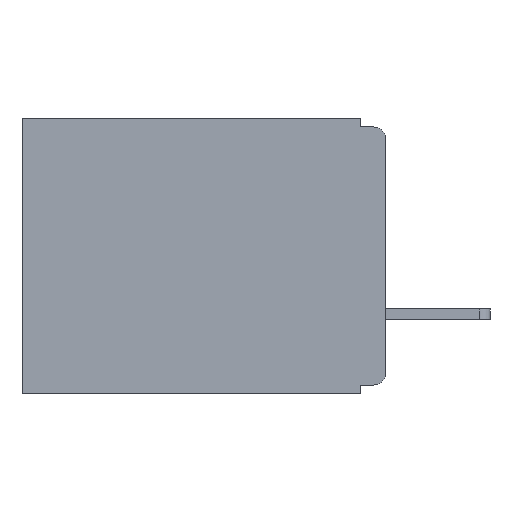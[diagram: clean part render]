
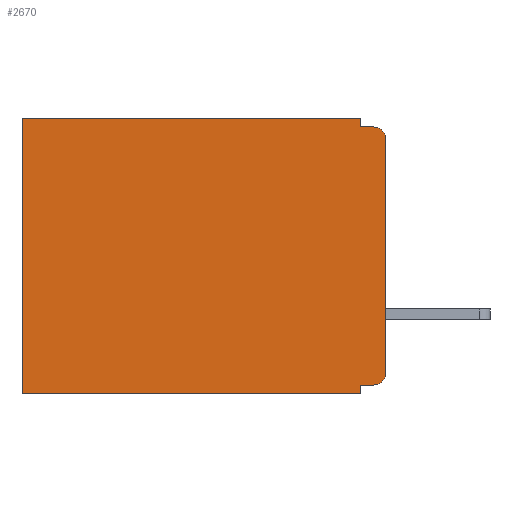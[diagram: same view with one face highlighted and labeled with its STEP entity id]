
A CAD part, left-side view. The second image highlights one B-rep face of the part: STEP entity #2670.
In plain terms, the highlighted planar face has unit normal (-1, 0, 0).
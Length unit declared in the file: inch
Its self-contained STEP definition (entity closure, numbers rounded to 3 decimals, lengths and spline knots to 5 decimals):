
#90 = DIRECTION ( 'NONE',  ( 0., 1., 0. ) ) ;
#333 = VERTEX_POINT ( 'NONE', #2948 ) ;
#765 = VERTEX_POINT ( 'NONE', #2917 ) ;
#828 = CARTESIAN_POINT ( 'NONE',  ( 0.3, 0., -0.025 ) ) ;
#943 = DIRECTION ( 'NONE',  ( 0., 0., -1. ) ) ;
#1069 = ORIENTED_EDGE ( 'NONE', *, *, #9149, .F. ) ;
#1142 = EDGE_CURVE ( 'NONE', #11783, #6901, #10360, .T. ) ;
#1357 = VERTEX_POINT ( 'NONE', #3417 ) ;
#1366 = VERTEX_POINT ( 'NONE', #7009 ) ;
#1420 = ORIENTED_EDGE ( 'NONE', *, *, #1142, .T. ) ;
#1744 = CIRCLE ( 'NONE', #13698, 0.015 ) ;
#1860 = DIRECTION ( 'NONE',  ( 1., 0., 0. ) ) ;
#1912 = CARTESIAN_POINT ( 'NONE',  ( 0.3, 0., -0.33 ) ) ;
#2081 = CARTESIAN_POINT ( 'NONE',  ( 0.3, 0., 0. ) ) ;
#2464 = ORIENTED_EDGE ( 'NONE', *, *, #17892, .T. ) ;
#2581 = DIRECTION ( 'NONE',  ( 0., 0., -1. ) ) ;
#2670 = ADVANCED_FACE ( 'NONE', ( #14872 ), #19481, .F. ) ;
#2890 = CARTESIAN_POINT ( 'NONE',  ( 0.3, 0., -0.33 ) ) ;
#2917 = CARTESIAN_POINT ( 'NONE',  ( 0.3, 0.015, -0.32 ) ) ;
#2948 = CARTESIAN_POINT ( 'NONE',  ( 0.3, 0.031, -0.32 ) ) ;
#3417 = CARTESIAN_POINT ( 'NONE',  ( 0.3, 0.031, 0. ) ) ;
#3494 = EDGE_CURVE ( 'NONE', #20158, #6901, #7287, .T. ) ;
#3505 = CARTESIAN_POINT ( 'NONE',  ( 0.3, 0.031, 0. ) ) ;
#3595 = CARTESIAN_POINT ( 'NONE',  ( 0.3, 0.437, 0. ) ) ;
#4510 = VECTOR ( 'NONE', #5199, 39.37008 ) ;
#4785 = ORIENTED_EDGE ( 'NONE', *, *, #3494, .F. ) ;
#4812 = CARTESIAN_POINT ( 'NONE',  ( 0.3, 0.031, -0.01 ) ) ;
#4928 = CARTESIAN_POINT ( 'NONE',  ( 0.3, 0.031, -0.33 ) ) ;
#4936 = ORIENTED_EDGE ( 'NONE', *, *, #19475, .F. ) ;
#5199 = DIRECTION ( 'NONE',  ( 0., 0., -1. ) ) ;
#5347 = DIRECTION ( 'NONE',  ( 0., 1., 0. ) ) ;
#6072 = VECTOR ( 'NONE', #14582, 39.37008 ) ;
#6260 = EDGE_CURVE ( 'NONE', #333, #11001, #10334, .T. ) ;
#6472 = CARTESIAN_POINT ( 'NONE',  ( 0.3, 0., -0.305 ) ) ;
#6576 = ORIENTED_EDGE ( 'NONE', *, *, #10588, .T. ) ;
#6644 = LINE ( 'NONE', #8546, #19457 ) ;
#6901 = VERTEX_POINT ( 'NONE', #19391 ) ;
#7009 = CARTESIAN_POINT ( 'NONE',  ( 0.3, 0.437, -0.33 ) ) ;
#7179 = LINE ( 'NONE', #2081, #19474 ) ;
#7287 = LINE ( 'NONE', #9218, #15340 ) ;
#8459 = LINE ( 'NONE', #13092, #20760 ) ;
#8546 = CARTESIAN_POINT ( 'NONE',  ( 0.3, 0., -0.33 ) ) ;
#9149 = EDGE_CURVE ( 'NONE', #765, #333, #8459, .T. ) ;
#9218 = CARTESIAN_POINT ( 'NONE',  ( 0.3, 0., -0.01 ) ) ;
#9881 = EDGE_CURVE ( 'NONE', #1357, #20459, #7179, .T. ) ;
#10145 = CARTESIAN_POINT ( 'NONE',  ( 0.3, 0.031, -0.33 ) ) ;
#10334 = LINE ( 'NONE', #4928, #6072 ) ;
#10360 = CIRCLE ( 'NONE', #13782, 0.015 ) ;
#10588 = EDGE_CURVE ( 'NONE', #765, #17858, #1744, .T. ) ;
#10680 = AXIS2_PLACEMENT_3D ( 'NONE', #1912, #1860, #2581 ) ;
#10712 = DIRECTION ( 'NONE',  ( -1., 0., 0. ) ) ;
#10807 = DIRECTION ( 'NONE',  ( 0., -1., 0. ) ) ;
#10984 = EDGE_CURVE ( 'NONE', #11001, #1366, #6644, .T. ) ;
#11001 = VERTEX_POINT ( 'NONE', #10145 ) ;
#11019 = EDGE_LOOP ( 'NONE', ( #4936, #1420, #4785, #15906, #15559, #2464, #15051, #19556, #1069, #6576 ) ) ;
#11372 = DIRECTION ( 'NONE',  ( 0., 0., -1. ) ) ;
#11783 = VERTEX_POINT ( 'NONE', #828 ) ;
#11834 = LINE ( 'NONE', #19397, #18912 ) ;
#12044 = LINE ( 'NONE', #2890, #16361 ) ;
#13092 = CARTESIAN_POINT ( 'NONE',  ( 0.3, 0., -0.32 ) ) ;
#13698 = AXIS2_PLACEMENT_3D ( 'NONE', #20350, #10712, #943 ) ;
#13782 = AXIS2_PLACEMENT_3D ( 'NONE', #18308, #18779, #20984 ) ;
#14582 = DIRECTION ( 'NONE',  ( 0., 0., -1. ) ) ;
#14872 = FACE_OUTER_BOUND ( 'NONE', #11019, .T. ) ;
#15051 = ORIENTED_EDGE ( 'NONE', *, *, #10984, .F. ) ;
#15340 = VECTOR ( 'NONE', #10807, 39.37008 ) ;
#15559 = ORIENTED_EDGE ( 'NONE', *, *, #9881, .T. ) ;
#15906 = ORIENTED_EDGE ( 'NONE', *, *, #17988, .F. ) ;
#16361 = VECTOR ( 'NONE', #20600, 39.37008 ) ;
#17406 = LINE ( 'NONE', #3505, #4510 ) ;
#17858 = VERTEX_POINT ( 'NONE', #6472 ) ;
#17892 = EDGE_CURVE ( 'NONE', #20459, #1366, #11834, .T. ) ;
#17988 = EDGE_CURVE ( 'NONE', #1357, #20158, #17406, .T. ) ;
#18308 = CARTESIAN_POINT ( 'NONE',  ( 0.3, 0.015, -0.025 ) ) ;
#18779 = DIRECTION ( 'NONE',  ( -1., 0., 0. ) ) ;
#18912 = VECTOR ( 'NONE', #11372, 39.37008 ) ;
#19391 = CARTESIAN_POINT ( 'NONE',  ( 0.3, 0.015, -0.01 ) ) ;
#19397 = CARTESIAN_POINT ( 'NONE',  ( 0.3, 0.437, -0.33 ) ) ;
#19457 = VECTOR ( 'NONE', #19778, 39.37008 ) ;
#19474 = VECTOR ( 'NONE', #5347, 39.37008 ) ;
#19475 = EDGE_CURVE ( 'NONE', #11783, #17858, #12044, .T. ) ;
#19481 = PLANE ( 'NONE',  #10680 ) ;
#19556 = ORIENTED_EDGE ( 'NONE', *, *, #6260, .F. ) ;
#19778 = DIRECTION ( 'NONE',  ( 0., 1., 0. ) ) ;
#20158 = VERTEX_POINT ( 'NONE', #4812 ) ;
#20350 = CARTESIAN_POINT ( 'NONE',  ( 0.3, 0.015, -0.305 ) ) ;
#20459 = VERTEX_POINT ( 'NONE', #3595 ) ;
#20600 = DIRECTION ( 'NONE',  ( 0., 0., -1. ) ) ;
#20760 = VECTOR ( 'NONE', #90, 39.37008 ) ;
#20984 = DIRECTION ( 'NONE',  ( 0., 0., -1. ) ) ;
